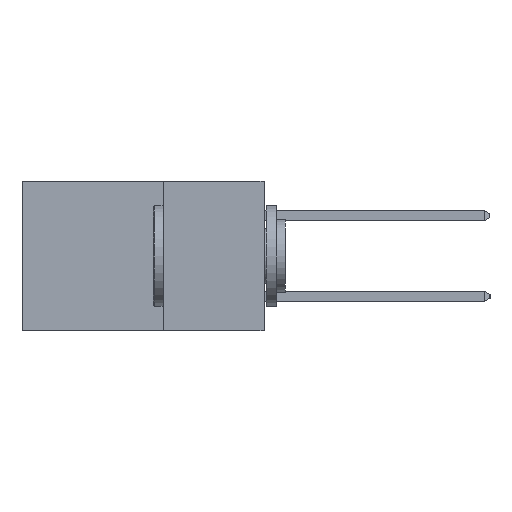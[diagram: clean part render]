
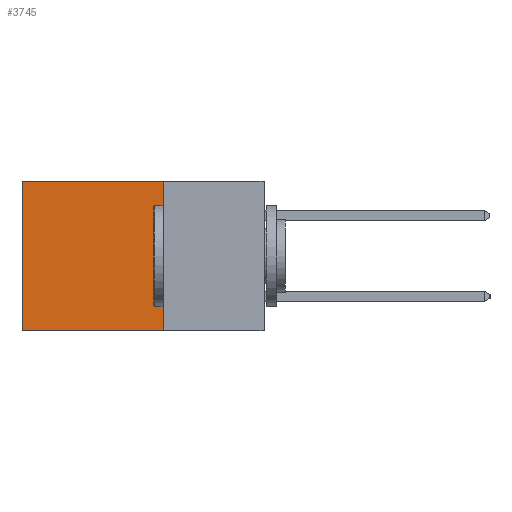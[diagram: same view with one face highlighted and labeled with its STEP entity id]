
A CAD part, left-side view. The second image highlights one B-rep face of the part: STEP entity #3745.
In plain terms, the highlighted planar face has unit normal (-1, 0, 0).
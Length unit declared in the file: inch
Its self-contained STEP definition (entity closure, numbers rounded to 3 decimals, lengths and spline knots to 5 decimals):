
#350 = CARTESIAN_POINT ( 'NONE',  ( 0.2615, 0.6, -0.37 ) ) ;
#462 = CARTESIAN_POINT ( 'NONE',  ( 0.2615, 0.6, -0.37 ) ) ;
#538 = VECTOR ( 'NONE', #8151, 39.37008 ) ;
#848 = LINE ( 'NONE', #12112, #10392 ) ;
#1304 = CARTESIAN_POINT ( 'NONE',  ( 0.2615, 0.25, 0. ) ) ;
#1335 = VERTEX_POINT ( 'NONE', #4093 ) ;
#1432 = ORIENTED_EDGE ( 'NONE', *, *, #2002, .F. ) ;
#2002 = EDGE_CURVE ( 'NONE', #4924, #1335, #10252, .T. ) ;
#2345 = CARTESIAN_POINT ( 'NONE',  ( 0.2615, 0.6, 0. ) ) ;
#2481 = DIRECTION ( 'NONE',  ( 0., 0., -1. ) ) ;
#2781 = ORIENTED_EDGE ( 'NONE', *, *, #10137, .T. ) ;
#3745 = ADVANCED_FACE ( 'NONE', ( #12169 ), #10031, .F. ) ;
#3776 = VERTEX_POINT ( 'NONE', #462 ) ;
#4032 = DIRECTION ( 'NONE',  ( 0., 1., 0. ) ) ;
#4060 = EDGE_LOOP ( 'NONE', ( #11939, #12027, #1432, #2781 ) ) ;
#4093 = CARTESIAN_POINT ( 'NONE',  ( 0.2615, 0.25, -0.37 ) ) ;
#4245 = AXIS2_PLACEMENT_3D ( 'NONE', #10928, #5517, #11776 ) ;
#4924 = VERTEX_POINT ( 'NONE', #1304 ) ;
#5517 = DIRECTION ( 'NONE',  ( 1., 0., 0. ) ) ;
#5586 = CARTESIAN_POINT ( 'NONE',  ( 0.2615, 0.25, -0.37 ) ) ;
#5840 = VECTOR ( 'NONE', #4032, 39.37008 ) ;
#6743 = EDGE_CURVE ( 'NONE', #1335, #3776, #8245, .T. ) ;
#8151 = DIRECTION ( 'NONE',  ( 0., 0., -1. ) ) ;
#8245 = LINE ( 'NONE', #10331, #5840 ) ;
#8321 = LINE ( 'NONE', #350, #538 ) ;
#8553 = DIRECTION ( 'NONE',  ( 0., 1., 0. ) ) ;
#9215 = EDGE_CURVE ( 'NONE', #9687, #3776, #8321, .T. ) ;
#9687 = VERTEX_POINT ( 'NONE', #2345 ) ;
#10031 = PLANE ( 'NONE',  #4245 ) ;
#10137 = EDGE_CURVE ( 'NONE', #4924, #9687, #848, .T. ) ;
#10252 = LINE ( 'NONE', #5586, #12009 ) ;
#10331 = CARTESIAN_POINT ( 'NONE',  ( 0.2615, 0.25, -0.37 ) ) ;
#10392 = VECTOR ( 'NONE', #8553, 39.37008 ) ;
#10928 = CARTESIAN_POINT ( 'NONE',  ( 0.2615, 0.25, -0.37 ) ) ;
#11776 = DIRECTION ( 'NONE',  ( 0., 0., -1. ) ) ;
#11939 = ORIENTED_EDGE ( 'NONE', *, *, #9215, .T. ) ;
#12009 = VECTOR ( 'NONE', #2481, 39.37008 ) ;
#12027 = ORIENTED_EDGE ( 'NONE', *, *, #6743, .F. ) ;
#12112 = CARTESIAN_POINT ( 'NONE',  ( 0.2615, 0.25, 0. ) ) ;
#12169 = FACE_OUTER_BOUND ( 'NONE', #4060, .T. ) ;
